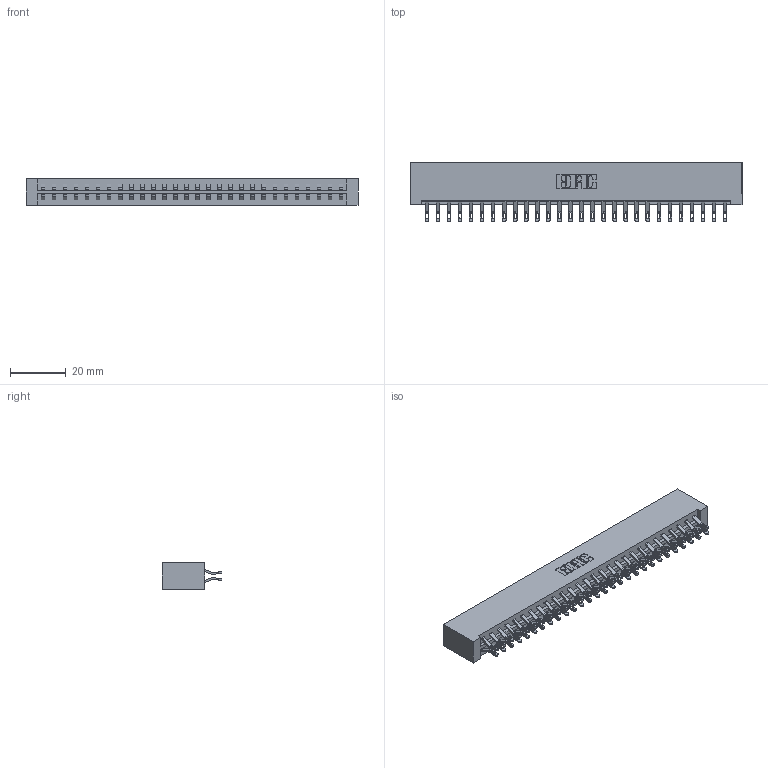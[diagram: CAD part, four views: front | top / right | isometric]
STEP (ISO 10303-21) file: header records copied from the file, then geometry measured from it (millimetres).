
FILE_DESCRIPTION (( 'STEP AP203' ), '1' );
FILE_NAME ('833-056-555-201.STEP', '2020-06-04T23:08:11', ( '' ), ( '' ), 'SwSTEP 2.0', 'SolidWorks 2020', '' );
FILE_SCHEMA (( 'CONFIG_CONTROL_DESIGN' ));
Length unit declared in the file: inch
Products named in the file (3): 833 Part_Lugless; 833-056-555-201; 345-292-001_555 Tail
Assembly tree (57 placements, depth 2):
  833-056-555-201
    833 Part_Lugless
    345-292-001_555 Tail  x56
Bounding box: 119.2 x 21.47 x 9.4 mm (x, y, z)
Volume: 12833.6 mm3; surface area: 15653.9 mm2
Topology: 57 solids, 57 shells, 3354 faces, 10535 edges, 7022 vertices
Faces by surface type: plane 1970, cylinder 1384
Entity records: 19873 total; most frequent: CARTESIAN_POINT 3344, ORIENTED_EDGE 3250, DIRECTION 2845, EDGE_CURVE 1625, LINE 1485, VECTOR 1485, VERTEX_POINT 1082, AXIS2_PLACEMENT_3D 680
